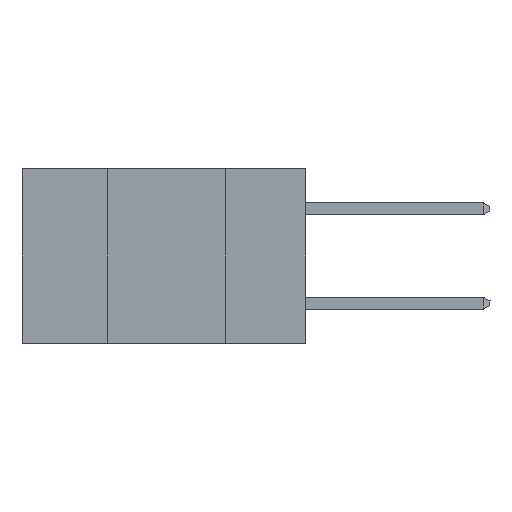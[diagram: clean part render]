
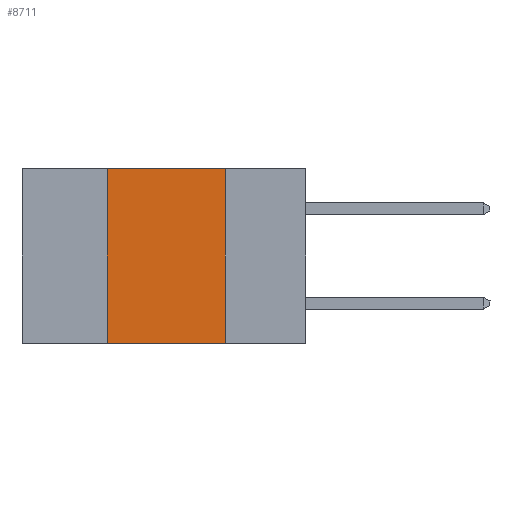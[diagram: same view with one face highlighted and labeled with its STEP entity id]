
A CAD part, left-side view. The second image highlights one B-rep face of the part: STEP entity #8711.
In plain terms, the highlighted planar face has unit normal (-1, 0, 0).
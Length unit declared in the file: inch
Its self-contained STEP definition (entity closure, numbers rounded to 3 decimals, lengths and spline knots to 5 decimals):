
#169 = PLANE ( 'NONE',  #3079 ) ;
#598 = VECTOR ( 'NONE', #11971, 39.37008 ) ;
#666 = LINE ( 'NONE', #11876, #7022 ) ;
#756 = EDGE_CURVE ( 'NONE', #13518, #17689, #12685, .T. ) ;
#993 = CARTESIAN_POINT ( 'NONE',  ( 0., 0.42, 0. ) ) ;
#1316 = VERTEX_POINT ( 'NONE', #15766 ) ;
#3079 = AXIS2_PLACEMENT_3D ( 'NONE', #12520, #11036, #4165 ) ;
#4069 = ORIENTED_EDGE ( 'NONE', *, *, #756, .F. ) ;
#4102 = DIRECTION ( 'NONE',  ( 0., 0., -1. ) ) ;
#4165 = DIRECTION ( 'NONE',  ( 0., 0., -1. ) ) ;
#4386 = VECTOR ( 'NONE', #15506, 39.37008 ) ;
#4536 = ORIENTED_EDGE ( 'NONE', *, *, #10900, .F. ) ;
#5012 = CARTESIAN_POINT ( 'NONE',  ( 0., 0.17, 0. ) ) ;
#5433 = VECTOR ( 'NONE', #4102, 39.37008 ) ;
#5565 = ORIENTED_EDGE ( 'NONE', *, *, #12026, .F. ) ;
#7022 = VECTOR ( 'NONE', #16020, 39.37008 ) ;
#7883 = EDGE_CURVE ( 'NONE', #13518, #1316, #8888, .T. ) ;
#8711 = ADVANCED_FACE ( 'NONE', ( #14233 ), #169, .F. ) ;
#8845 = LINE ( 'NONE', #15016, #5433 ) ;
#8888 = LINE ( 'NONE', #13950, #4386 ) ;
#10900 = EDGE_CURVE ( 'NONE', #17689, #11997, #666, .T. ) ;
#11036 = DIRECTION ( 'NONE',  ( 1., 0., 0. ) ) ;
#11876 = CARTESIAN_POINT ( 'NONE',  ( 0., 0.6, 0. ) ) ;
#11971 = DIRECTION ( 'NONE',  ( 0., 0., 1. ) ) ;
#11997 = VERTEX_POINT ( 'NONE', #5012 ) ;
#12026 = EDGE_CURVE ( 'NONE', #11997, #1316, #8845, .T. ) ;
#12520 = CARTESIAN_POINT ( 'NONE',  ( 0., 0.6, 0. ) ) ;
#12685 = LINE ( 'NONE', #993, #598 ) ;
#13518 = VERTEX_POINT ( 'NONE', #15201 ) ;
#13900 = CARTESIAN_POINT ( 'NONE',  ( 0., 0.42, 0. ) ) ;
#13950 = CARTESIAN_POINT ( 'NONE',  ( 0., 0.6, -0.37 ) ) ;
#14233 = FACE_OUTER_BOUND ( 'NONE', #17817, .T. ) ;
#14244 = ORIENTED_EDGE ( 'NONE', *, *, #7883, .T. ) ;
#15016 = CARTESIAN_POINT ( 'NONE',  ( 0., 0.17, 0. ) ) ;
#15201 = CARTESIAN_POINT ( 'NONE',  ( 0., 0.42, -0.37 ) ) ;
#15506 = DIRECTION ( 'NONE',  ( 0., -1., 0. ) ) ;
#15766 = CARTESIAN_POINT ( 'NONE',  ( 0., 0.17, -0.37 ) ) ;
#16020 = DIRECTION ( 'NONE',  ( 0., -1., 0. ) ) ;
#17689 = VERTEX_POINT ( 'NONE', #13900 ) ;
#17817 = EDGE_LOOP ( 'NONE', ( #5565, #4536, #4069, #14244 ) ) ;
